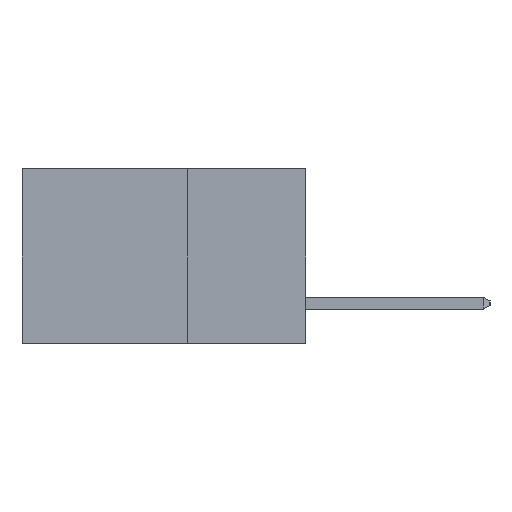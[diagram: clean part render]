
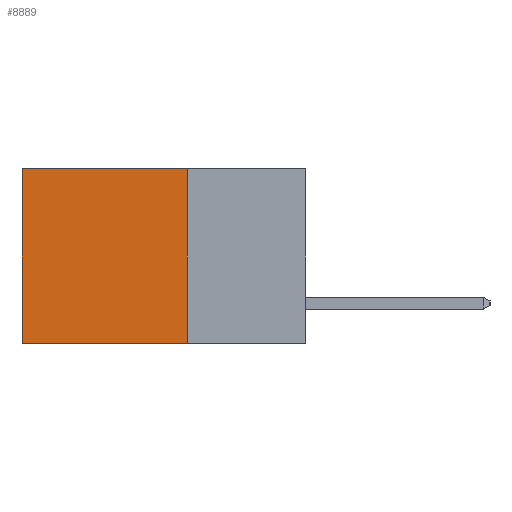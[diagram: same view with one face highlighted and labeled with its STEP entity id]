
A CAD part, left-side view. The second image highlights one B-rep face of the part: STEP entity #8889.
In plain terms, the highlighted planar face has unit normal (-1, 0, 0).
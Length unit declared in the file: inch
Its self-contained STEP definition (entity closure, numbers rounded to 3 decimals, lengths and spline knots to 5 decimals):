
#828 = ORIENTED_EDGE ( 'NONE', *, *, #3206, .F. ) ;
#1041 = AXIS2_PLACEMENT_3D ( 'NONE', #14882, #14814, #14796 ) ;
#1084 = VERTEX_POINT ( 'NONE', #8310 ) ;
#2056 = CARTESIAN_POINT ( 'NONE',  ( 0.2615, 0.6, -0.37 ) ) ;
#2210 = VECTOR ( 'NONE', #2319, 39.37008 ) ;
#2319 = DIRECTION ( 'NONE',  ( 0., 0., -1. ) ) ;
#2340 = CARTESIAN_POINT ( 'NONE',  ( 0.2615, 0.25, -0.37 ) ) ;
#2345 = CARTESIAN_POINT ( 'NONE',  ( 0.2615, 0.25, -0.37 ) ) ;
#3206 = EDGE_CURVE ( 'NONE', #16559, #6075, #11660, .T. ) ;
#3686 = ORIENTED_EDGE ( 'NONE', *, *, #10371, .F. ) ;
#4571 = EDGE_CURVE ( 'NONE', #1084, #5602, #17140, .T. ) ;
#5443 = VECTOR ( 'NONE', #6143, 39.37008 ) ;
#5602 = VERTEX_POINT ( 'NONE', #15867 ) ;
#5812 = FACE_OUTER_BOUND ( 'NONE', #11125, .T. ) ;
#6075 = VERTEX_POINT ( 'NONE', #2056 ) ;
#6143 = DIRECTION ( 'NONE',  ( 0., 0., -1. ) ) ;
#6327 = CARTESIAN_POINT ( 'NONE',  ( 0.2615, 0.6, -0.37 ) ) ;
#7208 = EDGE_CURVE ( 'NONE', #5602, #6075, #16446, .T. ) ;
#7958 = VECTOR ( 'NONE', #8128, 39.37008 ) ;
#8128 = DIRECTION ( 'NONE',  ( 0., 1., 0. ) ) ;
#8310 = CARTESIAN_POINT ( 'NONE',  ( 0.2615, 0.25, 0. ) ) ;
#8507 = ORIENTED_EDGE ( 'NONE', *, *, #7208, .T. ) ;
#8889 = ADVANCED_FACE ( 'NONE', ( #5812 ), #14857, .F. ) ;
#9860 = VECTOR ( 'NONE', #14037, 39.37008 ) ;
#10371 = EDGE_CURVE ( 'NONE', #1084, #16559, #16937, .T. ) ;
#11125 = EDGE_LOOP ( 'NONE', ( #8507, #828, #3686, #15713 ) ) ;
#11660 = LINE ( 'NONE', #13930, #7958 ) ;
#13930 = CARTESIAN_POINT ( 'NONE',  ( 0.2615, 0.25, -0.37 ) ) ;
#14037 = DIRECTION ( 'NONE',  ( 0., 1., 0. ) ) ;
#14796 = DIRECTION ( 'NONE',  ( 0., 0., -1. ) ) ;
#14814 = DIRECTION ( 'NONE',  ( 1., 0., 0. ) ) ;
#14857 = PLANE ( 'NONE',  #1041 ) ;
#14882 = CARTESIAN_POINT ( 'NONE',  ( 0.2615, 0.25, -0.37 ) ) ;
#15713 = ORIENTED_EDGE ( 'NONE', *, *, #4571, .T. ) ;
#15867 = CARTESIAN_POINT ( 'NONE',  ( 0.2615, 0.6, 0. ) ) ;
#16208 = CARTESIAN_POINT ( 'NONE',  ( 0.2615, 0.25, 0. ) ) ;
#16446 = LINE ( 'NONE', #6327, #5443 ) ;
#16559 = VERTEX_POINT ( 'NONE', #2345 ) ;
#16937 = LINE ( 'NONE', #2340, #2210 ) ;
#17140 = LINE ( 'NONE', #16208, #9860 ) ;
